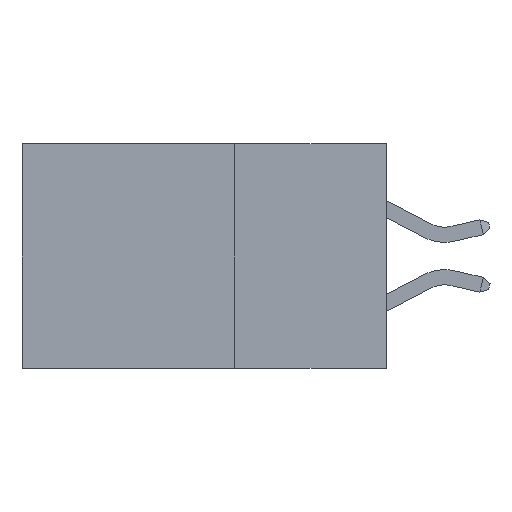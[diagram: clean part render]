
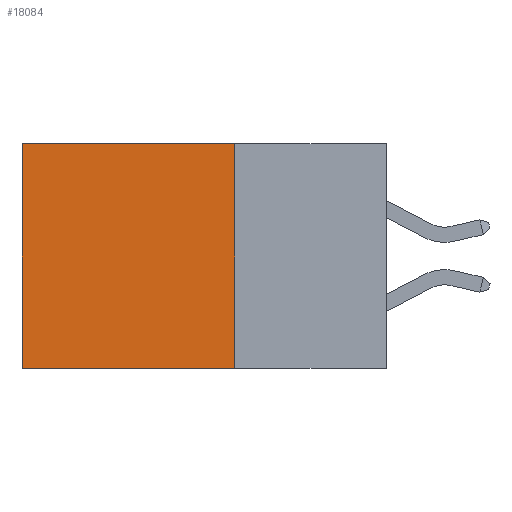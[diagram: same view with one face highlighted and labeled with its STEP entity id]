
A CAD part, left-side view. The second image highlights one B-rep face of the part: STEP entity #18084.
In plain terms, the highlighted planar face has unit normal (-1, 0, 0).
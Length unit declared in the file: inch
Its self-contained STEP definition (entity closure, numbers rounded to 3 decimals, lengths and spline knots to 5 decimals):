
#413 = EDGE_CURVE ( 'NONE', #6087, #5578, #893, .T. ) ;
#893 = LINE ( 'NONE', #10796, #13496 ) ;
#2285 = CARTESIAN_POINT ( 'NONE',  ( 0.2615, 0.25, -0.37 ) ) ;
#3394 = VECTOR ( 'NONE', #13650, 39.37008 ) ;
#3404 = CARTESIAN_POINT ( 'NONE',  ( 0.2615, 0.25, -0.37 ) ) ;
#3571 = CARTESIAN_POINT ( 'NONE',  ( 0.2615, 0.6, 0. ) ) ;
#3620 = CARTESIAN_POINT ( 'NONE',  ( 0.2615, 0.6, -0.37 ) ) ;
#3767 = AXIS2_PLACEMENT_3D ( 'NONE', #14677, #17937, #8272 ) ;
#4311 = VECTOR ( 'NONE', #7692, 39.37008 ) ;
#5578 = VERTEX_POINT ( 'NONE', #3404 ) ;
#5817 = FACE_OUTER_BOUND ( 'NONE', #15154, .T. ) ;
#6087 = VERTEX_POINT ( 'NONE', #13334 ) ;
#6373 = LINE ( 'NONE', #3620, #13946 ) ;
#6754 = CARTESIAN_POINT ( 'NONE',  ( 0.2615, 0.6, -0.37 ) ) ;
#7692 = DIRECTION ( 'NONE',  ( 0., 1., 0. ) ) ;
#7888 = ORIENTED_EDGE ( 'NONE', *, *, #11887, .T. ) ;
#8272 = DIRECTION ( 'NONE',  ( 0., 0., -1. ) ) ;
#9165 = EDGE_CURVE ( 'NONE', #5578, #12271, #16334, .T. ) ;
#10796 = CARTESIAN_POINT ( 'NONE',  ( 0.2615, 0.25, -0.37 ) ) ;
#10859 = EDGE_CURVE ( 'NONE', #15257, #12271, #6373, .T. ) ;
#11887 = EDGE_CURVE ( 'NONE', #6087, #15257, #12443, .T. ) ;
#11906 = ORIENTED_EDGE ( 'NONE', *, *, #9165, .F. ) ;
#12271 = VERTEX_POINT ( 'NONE', #6754 ) ;
#12443 = LINE ( 'NONE', #12528, #4311 ) ;
#12528 = CARTESIAN_POINT ( 'NONE',  ( 0.2615, 0.25, 0. ) ) ;
#13077 = PLANE ( 'NONE',  #3767 ) ;
#13334 = CARTESIAN_POINT ( 'NONE',  ( 0.2615, 0.25, 0. ) ) ;
#13496 = VECTOR ( 'NONE', #15403, 39.37008 ) ;
#13650 = DIRECTION ( 'NONE',  ( 0., 1., 0. ) ) ;
#13862 = ORIENTED_EDGE ( 'NONE', *, *, #10859, .T. ) ;
#13946 = VECTOR ( 'NONE', #16581, 39.37008 ) ;
#14677 = CARTESIAN_POINT ( 'NONE',  ( 0.2615, 0.25, -0.37 ) ) ;
#15154 = EDGE_LOOP ( 'NONE', ( #13862, #11906, #18156, #7888 ) ) ;
#15257 = VERTEX_POINT ( 'NONE', #3571 ) ;
#15403 = DIRECTION ( 'NONE',  ( 0., 0., -1. ) ) ;
#16334 = LINE ( 'NONE', #2285, #3394 ) ;
#16581 = DIRECTION ( 'NONE',  ( 0., 0., -1. ) ) ;
#17937 = DIRECTION ( 'NONE',  ( 1., 0., 0. ) ) ;
#18084 = ADVANCED_FACE ( 'NONE', ( #5817 ), #13077, .F. ) ;
#18156 = ORIENTED_EDGE ( 'NONE', *, *, #413, .F. ) ;
